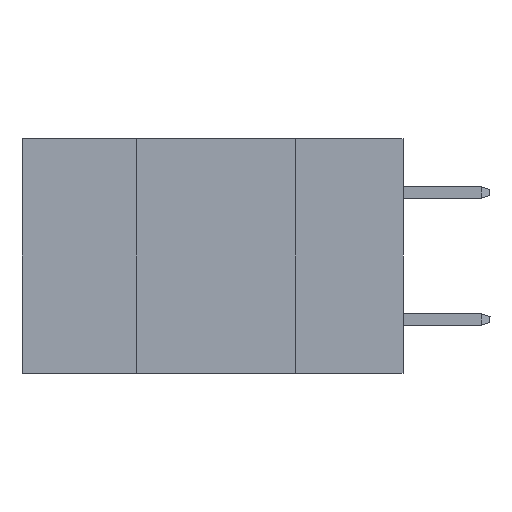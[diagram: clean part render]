
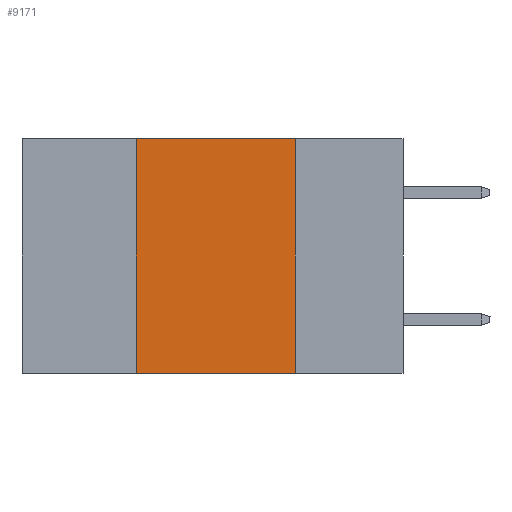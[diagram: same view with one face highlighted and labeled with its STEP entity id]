
A CAD part, left-side view. The second image highlights one B-rep face of the part: STEP entity #9171.
In plain terms, the highlighted planar face has unit normal (-1, 0, 0).
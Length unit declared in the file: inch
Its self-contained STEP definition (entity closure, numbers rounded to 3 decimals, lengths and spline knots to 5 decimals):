
#858 = CARTESIAN_POINT ( 'NONE',  ( 0., 0.6, 0. ) ) ;
#1484 = DIRECTION ( 'NONE',  ( 0., 0., -1. ) ) ;
#2742 = ORIENTED_EDGE ( 'NONE', *, *, #25389, .F. ) ;
#4025 = VERTEX_POINT ( 'NONE', #11632 ) ;
#5158 = EDGE_LOOP ( 'NONE', ( #30319, #2742, #26730, #19420 ) ) ;
#6527 = CARTESIAN_POINT ( 'NONE',  ( 0., 0.42, 0. ) ) ;
#9171 = ADVANCED_FACE ( 'NONE', ( #26946 ), #30798, .F. ) ;
#10548 = EDGE_CURVE ( 'NONE', #4025, #24331, #35279, .T. ) ;
#11166 = VERTEX_POINT ( 'NONE', #6527 ) ;
#11632 = CARTESIAN_POINT ( 'NONE',  ( 0., 0.17, 0. ) ) ;
#13597 = VECTOR ( 'NONE', #14239, 39.37008 ) ;
#14239 = DIRECTION ( 'NONE',  ( 0., -1., 0. ) ) ;
#15643 = LINE ( 'NONE', #18874, #19620 ) ;
#17438 = CARTESIAN_POINT ( 'NONE',  ( 0., 0.6, 0. ) ) ;
#18050 = VECTOR ( 'NONE', #27694, 39.37008 ) ;
#18449 = EDGE_CURVE ( 'NONE', #29864, #24331, #37582, .T. ) ;
#18874 = CARTESIAN_POINT ( 'NONE',  ( 0., 0.42, 0. ) ) ;
#19420 = ORIENTED_EDGE ( 'NONE', *, *, #18449, .T. ) ;
#19620 = VECTOR ( 'NONE', #34722, 39.37008 ) ;
#20481 = LINE ( 'NONE', #17438, #13597 ) ;
#20491 = VECTOR ( 'NONE', #25430, 39.37008 ) ;
#21922 = CARTESIAN_POINT ( 'NONE',  ( 0., 0.42, -0.37 ) ) ;
#22013 = CARTESIAN_POINT ( 'NONE',  ( 0., 0.17, 0. ) ) ;
#24308 = CARTESIAN_POINT ( 'NONE',  ( 0., 0.6, -0.37 ) ) ;
#24331 = VERTEX_POINT ( 'NONE', #41904 ) ;
#25389 = EDGE_CURVE ( 'NONE', #11166, #4025, #20481, .T. ) ;
#25430 = DIRECTION ( 'NONE',  ( 0., 0., -1. ) ) ;
#26730 = ORIENTED_EDGE ( 'NONE', *, *, #31636, .F. ) ;
#26946 = FACE_OUTER_BOUND ( 'NONE', #5158, .T. ) ;
#27694 = DIRECTION ( 'NONE',  ( 0., -1., 0. ) ) ;
#29864 = VERTEX_POINT ( 'NONE', #21922 ) ;
#30319 = ORIENTED_EDGE ( 'NONE', *, *, #10548, .F. ) ;
#30798 = PLANE ( 'NONE',  #36818 ) ;
#31636 = EDGE_CURVE ( 'NONE', #29864, #11166, #15643, .T. ) ;
#34722 = DIRECTION ( 'NONE',  ( 0., 0., 1. ) ) ;
#35279 = LINE ( 'NONE', #22013, #20491 ) ;
#36818 = AXIS2_PLACEMENT_3D ( 'NONE', #858, #40452, #1484 ) ;
#37582 = LINE ( 'NONE', #24308, #18050 ) ;
#40452 = DIRECTION ( 'NONE',  ( 1., 0., 0. ) ) ;
#41904 = CARTESIAN_POINT ( 'NONE',  ( 0., 0.17, -0.37 ) ) ;
